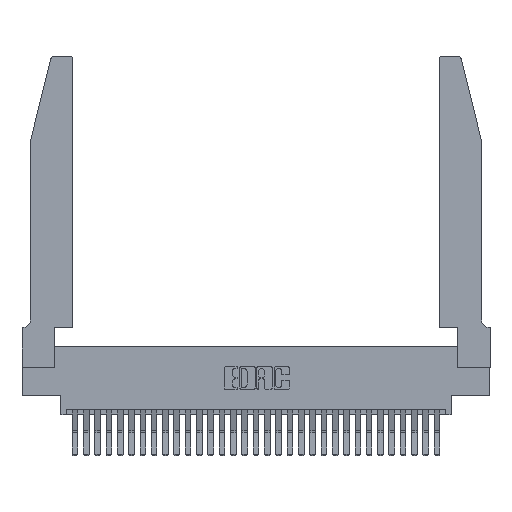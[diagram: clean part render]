
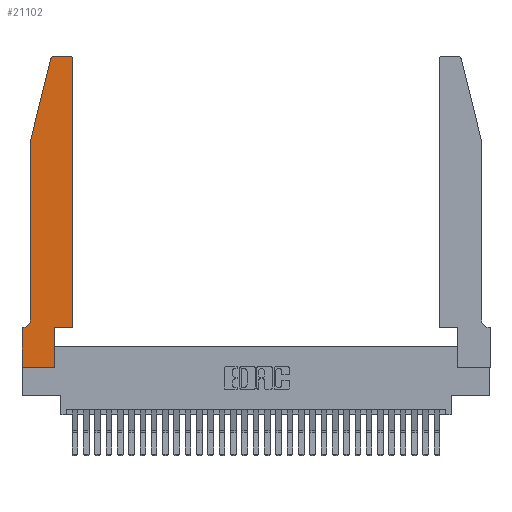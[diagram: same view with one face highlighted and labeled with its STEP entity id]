
A CAD part, top view. The second image highlights one B-rep face of the part: STEP entity #21102.
In plain terms, the highlighted planar face has unit normal (0, 0, 1).
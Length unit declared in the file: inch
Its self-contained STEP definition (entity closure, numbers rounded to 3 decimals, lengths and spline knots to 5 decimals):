
#561 = CIRCLE ( 'NONE', #25670, 0.03 ) ;
#1104 = DIRECTION ( 'NONE',  ( 0., -1., 0. ) ) ;
#1200 = CARTESIAN_POINT ( 'NONE',  ( 0.0755, 2., 0.37 ) ) ;
#1327 = VERTEX_POINT ( 'NONE', #13994 ) ;
#1333 = EDGE_CURVE ( 'NONE', #23942, #22117, #29021, .T. ) ;
#2156 = LINE ( 'NONE', #11783, #19264 ) ;
#2369 = CARTESIAN_POINT ( 'NONE',  ( 0.4505, 0.35, 0.37 ) ) ;
#2636 = DIRECTION ( 'NONE',  ( 0., 0., 1. ) ) ;
#2889 = AXIS2_PLACEMENT_3D ( 'NONE', #7671, #3658, #18653 ) ;
#2918 = LINE ( 'NONE', #18274, #6040 ) ;
#3008 = CARTESIAN_POINT ( 'NONE',  ( 0.284, 2.75, 0.37 ) ) ;
#3031 = DIRECTION ( 'NONE',  ( -1., 0., 0. ) ) ;
#3390 = CARTESIAN_POINT ( 'NONE',  ( 0.0755, 0.42, 0.37 ) ) ;
#3498 = EDGE_CURVE ( 'NONE', #8339, #13201, #13745, .T. ) ;
#3514 = CARTESIAN_POINT ( 'NONE',  ( 0., 0., 0.37 ) ) ;
#3658 = DIRECTION ( 'NONE',  ( 0., 0., 1. ) ) ;
#4022 = EDGE_LOOP ( 'NONE', ( #28309, #15633, #21270, #15850, #9507, #19130, #14951, #13878, #19704, #8084, #14619, #29082 ) ) ;
#4891 = CARTESIAN_POINT ( 'NONE',  ( 0., 0.35, 0.37 ) ) ;
#4958 = DIRECTION ( 'NONE',  ( -1., 0., 0. ) ) ;
#5178 = CARTESIAN_POINT ( 'NONE',  ( 0.2865, 0.35, 0.37 ) ) ;
#5326 = CARTESIAN_POINT ( 'NONE',  ( 0.2865, 0.35, 0.37 ) ) ;
#6040 = VECTOR ( 'NONE', #1104, 39.37008 ) ;
#6928 = LINE ( 'NONE', #30338, #25916 ) ;
#7671 = CARTESIAN_POINT ( 'NONE',  ( 0.284, 2.72, 0.37 ) ) ;
#7790 = VERTEX_POINT ( 'NONE', #14677 ) ;
#8084 = ORIENTED_EDGE ( 'NONE', *, *, #25325, .T. ) ;
#8339 = VERTEX_POINT ( 'NONE', #3008 ) ;
#8449 = CIRCLE ( 'NONE', #23557, 0.07 ) ;
#9507 = ORIENTED_EDGE ( 'NONE', *, *, #25176, .T. ) ;
#9549 = EDGE_CURVE ( 'NONE', #1327, #8339, #2156, .T. ) ;
#9734 = EDGE_CURVE ( 'NONE', #28628, #18713, #2918, .T. ) ;
#9984 = CARTESIAN_POINT ( 'NONE',  ( 0., 0., 0.37 ) ) ;
#10217 = PLANE ( 'NONE',  #31976 ) ;
#10299 = DIRECTION ( 'NONE',  ( 0., 0., -1. ) ) ;
#10615 = CARTESIAN_POINT ( 'NONE',  ( 0., 0., 0.37 ) ) ;
#11018 = CARTESIAN_POINT ( 'NONE',  ( 0.2865, 0., 0.37 ) ) ;
#11783 = CARTESIAN_POINT ( 'NONE',  ( 0.2605, 2.75, 0.37 ) ) ;
#11798 = CARTESIAN_POINT ( 'NONE',  ( 0.0755, 2., 0.37 ) ) ;
#12718 = EDGE_CURVE ( 'NONE', #30079, #7790, #30618, .T. ) ;
#12804 = DIRECTION ( 'NONE',  ( 0., 0., 1. ) ) ;
#13201 = VERTEX_POINT ( 'NONE', #27995 ) ;
#13745 = CIRCLE ( 'NONE', #2889, 0.03 ) ;
#13872 = VECTOR ( 'NONE', #25789, 39.37008 ) ;
#13878 = ORIENTED_EDGE ( 'NONE', *, *, #31993, .T. ) ;
#13994 = CARTESIAN_POINT ( 'NONE',  ( 0.4205, 2.75, 0.37 ) ) ;
#14340 = VECTOR ( 'NONE', #20059, 39.37008 ) ;
#14488 = VERTEX_POINT ( 'NONE', #9984 ) ;
#14619 = ORIENTED_EDGE ( 'NONE', *, *, #12718, .T. ) ;
#14677 = CARTESIAN_POINT ( 'NONE',  ( 0.4505, 2.72, 0.37 ) ) ;
#14951 = ORIENTED_EDGE ( 'NONE', *, *, #17268, .T. ) ;
#15389 = CARTESIAN_POINT ( 'NONE',  ( 0.0055, 0.42, 0.37 ) ) ;
#15633 = ORIENTED_EDGE ( 'NONE', *, *, #3498, .T. ) ;
#15678 = LINE ( 'NONE', #1200, #16839 ) ;
#15736 = DIRECTION ( 'NONE',  ( -0.239, -0.971, 0. ) ) ;
#15850 = ORIENTED_EDGE ( 'NONE', *, *, #9734, .T. ) ;
#15940 = EDGE_CURVE ( 'NONE', #7790, #1327, #561, .T. ) ;
#16078 = LINE ( 'NONE', #10615, #29963 ) ;
#16839 = VECTOR ( 'NONE', #15736, 39.37008 ) ;
#17268 = EDGE_CURVE ( 'NONE', #21527, #14488, #16078, .T. ) ;
#17427 = EDGE_CURVE ( 'NONE', #13201, #28628, #15678, .T. ) ;
#17577 = VERTEX_POINT ( 'NONE', #31429 ) ;
#18274 = CARTESIAN_POINT ( 'NONE',  ( 0.0755, 2., 0.37 ) ) ;
#18653 = DIRECTION ( 'NONE',  ( 1., 0., 0. ) ) ;
#18713 = VERTEX_POINT ( 'NONE', #3390 ) ;
#19130 = ORIENTED_EDGE ( 'NONE', *, *, #25413, .T. ) ;
#19264 = VECTOR ( 'NONE', #4958, 39.37008 ) ;
#19704 = ORIENTED_EDGE ( 'NONE', *, *, #1333, .T. ) ;
#20059 = DIRECTION ( 'NONE',  ( 0., 1., 0. ) ) ;
#20131 = CARTESIAN_POINT ( 'NONE',  ( 0.4205, 2.72, 0.37 ) ) ;
#20317 = CARTESIAN_POINT ( 'NONE',  ( 0.4505, 0.35, 0.37 ) ) ;
#20531 = DIRECTION ( 'NONE',  ( 1., 0., 0. ) ) ;
#20905 = DIRECTION ( 'NONE',  ( 1., 0., 0. ) ) ;
#21102 = ADVANCED_FACE ( 'NONE', ( #29359 ), #10217, .T. ) ;
#21270 = ORIENTED_EDGE ( 'NONE', *, *, #17427, .T. ) ;
#21527 = VERTEX_POINT ( 'NONE', #4891 ) ;
#21713 = VECTOR ( 'NONE', #20531, 39.37008 ) ;
#22117 = VERTEX_POINT ( 'NONE', #5178 ) ;
#22519 = DIRECTION ( 'NONE',  ( 1., 0., 0. ) ) ;
#23298 = VECTOR ( 'NONE', #20905, 39.37008 ) ;
#23557 = AXIS2_PLACEMENT_3D ( 'NONE', #15389, #10299, #3031 ) ;
#23942 = VERTEX_POINT ( 'NONE', #11018 ) ;
#25071 = DIRECTION ( 'NONE',  ( 1., 0., 0. ) ) ;
#25176 = EDGE_CURVE ( 'NONE', #18713, #17577, #8449, .T. ) ;
#25325 = EDGE_CURVE ( 'NONE', #22117, #30079, #28235, .T. ) ;
#25413 = EDGE_CURVE ( 'NONE', #17577, #21527, #6928, .T. ) ;
#25670 = AXIS2_PLACEMENT_3D ( 'NONE', #20131, #2636, #22519 ) ;
#25789 = DIRECTION ( 'NONE',  ( 0., 1., 0. ) ) ;
#25916 = VECTOR ( 'NONE', #30753, 39.37008 ) ;
#27225 = CARTESIAN_POINT ( 'NONE',  ( 0.4505, 0.35, 0.37 ) ) ;
#27644 = CARTESIAN_POINT ( 'NONE',  ( 0., 0.35, 0.37 ) ) ;
#27995 = CARTESIAN_POINT ( 'NONE',  ( 0.25487, 2.72718, 0.37 ) ) ;
#28235 = LINE ( 'NONE', #20317, #21713 ) ;
#28309 = ORIENTED_EDGE ( 'NONE', *, *, #9549, .T. ) ;
#28628 = VERTEX_POINT ( 'NONE', #11798 ) ;
#29021 = LINE ( 'NONE', #5326, #13872 ) ;
#29082 = ORIENTED_EDGE ( 'NONE', *, *, #15940, .T. ) ;
#29359 = FACE_OUTER_BOUND ( 'NONE', #4022, .T. ) ;
#29963 = VECTOR ( 'NONE', #30035, 39.37008 ) ;
#30035 = DIRECTION ( 'NONE',  ( 0., -1., 0. ) ) ;
#30079 = VERTEX_POINT ( 'NONE', #27225 ) ;
#30338 = CARTESIAN_POINT ( 'NONE',  ( 0.0755, 0.35, 0.37 ) ) ;
#30616 = LINE ( 'NONE', #3514, #23298 ) ;
#30618 = LINE ( 'NONE', #2369, #14340 ) ;
#30753 = DIRECTION ( 'NONE',  ( -1., 0., 0. ) ) ;
#31429 = CARTESIAN_POINT ( 'NONE',  ( 0.0055, 0.35, 0.37 ) ) ;
#31976 = AXIS2_PLACEMENT_3D ( 'NONE', #27644, #12804, #25071 ) ;
#31993 = EDGE_CURVE ( 'NONE', #14488, #23942, #30616, .T. ) ;
